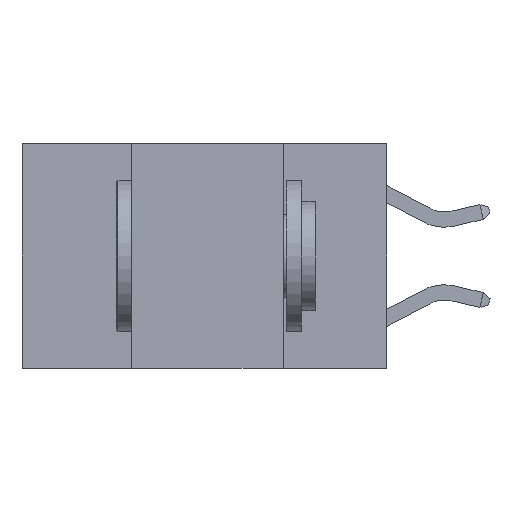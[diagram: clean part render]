
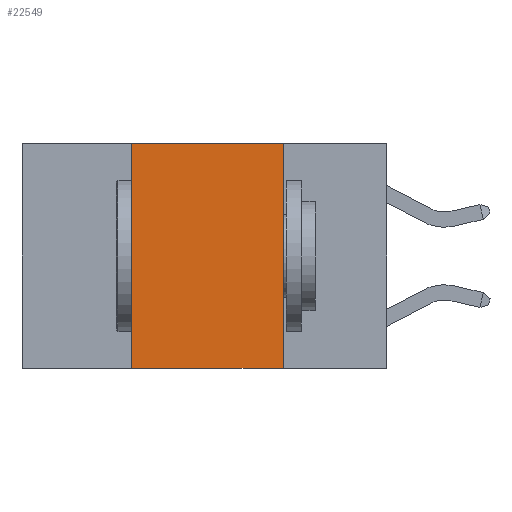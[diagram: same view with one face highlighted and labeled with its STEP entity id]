
A CAD part, left-side view. The second image highlights one B-rep face of the part: STEP entity #22549.
In plain terms, the highlighted planar face has unit normal (-1, 0, 0).
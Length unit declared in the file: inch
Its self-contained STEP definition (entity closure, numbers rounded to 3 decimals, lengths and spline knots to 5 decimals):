
#65 = ORIENTED_EDGE ( 'NONE', *, *, #10992, .F. ) ;
#70 = EDGE_CURVE ( 'NONE', #13087, #5910, #8727, .T. ) ;
#1522 = ORIENTED_EDGE ( 'NONE', *, *, #6438, .F. ) ;
#3330 = EDGE_CURVE ( 'NONE', #26931, #5910, #26643, .T. ) ;
#4675 = LINE ( 'NONE', #22473, #10113 ) ;
#5870 = CARTESIAN_POINT ( 'NONE',  ( 0., 0.6, -0.37 ) ) ;
#5910 = VERTEX_POINT ( 'NONE', #18642 ) ;
#6046 = LINE ( 'NONE', #11292, #11488 ) ;
#6438 = EDGE_CURVE ( 'NONE', #13087, #23860, #4675, .T. ) ;
#6708 = DIRECTION ( 'NONE',  ( 0., -1., 0. ) ) ;
#7560 = CARTESIAN_POINT ( 'NONE',  ( 0., 0.42, -0.37 ) ) ;
#7640 = ORIENTED_EDGE ( 'NONE', *, *, #70, .T. ) ;
#7987 = VECTOR ( 'NONE', #25579, 39.37008 ) ;
#8123 = DIRECTION ( 'NONE',  ( 0., 0., -1. ) ) ;
#8528 = VECTOR ( 'NONE', #8123, 39.37008 ) ;
#8727 = LINE ( 'NONE', #5870, #7987 ) ;
#10113 = VECTOR ( 'NONE', #17932, 39.37008 ) ;
#10964 = PLANE ( 'NONE',  #22976 ) ;
#10992 = EDGE_CURVE ( 'NONE', #23860, #26931, #6046, .T. ) ;
#11292 = CARTESIAN_POINT ( 'NONE',  ( 0., 0.6, 0. ) ) ;
#11488 = VECTOR ( 'NONE', #6708, 39.37008 ) ;
#13087 = VERTEX_POINT ( 'NONE', #7560 ) ;
#13846 = FACE_OUTER_BOUND ( 'NONE', #19225, .T. ) ;
#15561 = DIRECTION ( 'NONE',  ( 0., 0., -1. ) ) ;
#17932 = DIRECTION ( 'NONE',  ( 0., 0., 1. ) ) ;
#18642 = CARTESIAN_POINT ( 'NONE',  ( 0., 0.17, -0.37 ) ) ;
#19225 = EDGE_LOOP ( 'NONE', ( #27537, #65, #1522, #7640 ) ) ;
#19535 = CARTESIAN_POINT ( 'NONE',  ( 0., 0.17, 0. ) ) ;
#22473 = CARTESIAN_POINT ( 'NONE',  ( 0., 0.42, 0. ) ) ;
#22549 = ADVANCED_FACE ( 'NONE', ( #13846 ), #10964, .F. ) ;
#22976 = AXIS2_PLACEMENT_3D ( 'NONE', #26794, #29034, #15561 ) ;
#23860 = VERTEX_POINT ( 'NONE', #29252 ) ;
#25579 = DIRECTION ( 'NONE',  ( 0., -1., 0. ) ) ;
#26313 = CARTESIAN_POINT ( 'NONE',  ( 0., 0.17, 0. ) ) ;
#26643 = LINE ( 'NONE', #26313, #8528 ) ;
#26794 = CARTESIAN_POINT ( 'NONE',  ( 0., 0.6, 0. ) ) ;
#26931 = VERTEX_POINT ( 'NONE', #19535 ) ;
#27537 = ORIENTED_EDGE ( 'NONE', *, *, #3330, .F. ) ;
#29034 = DIRECTION ( 'NONE',  ( 1., 0., 0. ) ) ;
#29252 = CARTESIAN_POINT ( 'NONE',  ( 0., 0.42, 0. ) ) ;
